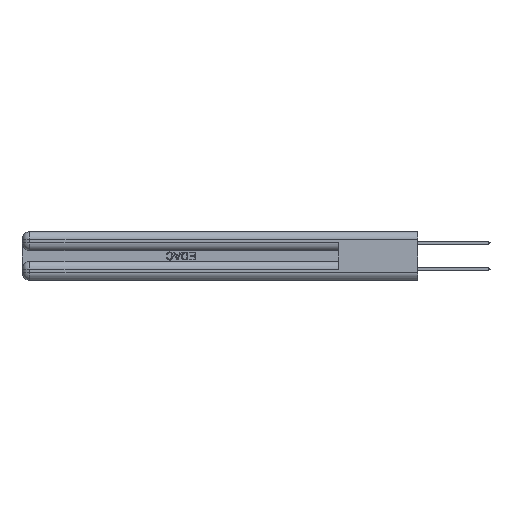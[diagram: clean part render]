
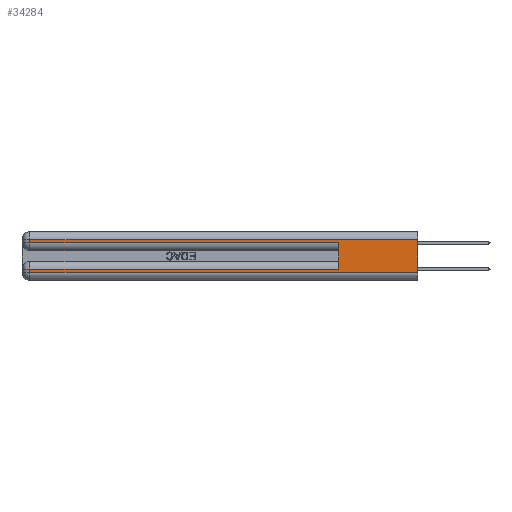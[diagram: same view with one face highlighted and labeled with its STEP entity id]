
A CAD part, left-side view. The second image highlights one B-rep face of the part: STEP entity #34284.
In plain terms, the highlighted planar face has unit normal (-1, 0, 0).
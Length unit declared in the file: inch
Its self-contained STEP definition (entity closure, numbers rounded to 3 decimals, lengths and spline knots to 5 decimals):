
#459 = DIRECTION ( 'NONE',  ( 0., 0., -1. ) ) ;
#741 = CARTESIAN_POINT ( 'NONE',  ( 0., 2.94, 0.31 ) ) ;
#1753 = DIRECTION ( 'NONE',  ( 0., -1., 0. ) ) ;
#1920 = DIRECTION ( 'NONE',  ( 0., 1., 0. ) ) ;
#2274 = VECTOR ( 'NONE', #1920, 39.37008 ) ;
#2917 = CARTESIAN_POINT ( 'NONE',  ( 0., 0., 0.31 ) ) ;
#3587 = CARTESIAN_POINT ( 'NONE',  ( 0., 0., 0.37 ) ) ;
#4552 = LINE ( 'NONE', #31151, #2274 ) ;
#6054 = VERTEX_POINT ( 'NONE', #741 ) ;
#6166 = ORIENTED_EDGE ( 'NONE', *, *, #24163, .F. ) ;
#6481 = EDGE_CURVE ( 'NONE', #37603, #10465, #30881, .T. ) ;
#7422 = VERTEX_POINT ( 'NONE', #20248 ) ;
#7532 = ORIENTED_EDGE ( 'NONE', *, *, #6481, .T. ) ;
#7965 = EDGE_CURVE ( 'NONE', #44316, #7422, #21030, .T. ) ;
#8741 = CARTESIAN_POINT ( 'NONE',  ( 0., 0., 0.06 ) ) ;
#8905 = DIRECTION ( 'NONE',  ( 0., 0., -1. ) ) ;
#9258 = ORIENTED_EDGE ( 'NONE', *, *, #30549, .T. ) ;
#10465 = VERTEX_POINT ( 'NONE', #8741 ) ;
#10579 = AXIS2_PLACEMENT_3D ( 'NONE', #35057, #38712, #16805 ) ;
#10701 = EDGE_CURVE ( 'NONE', #11947, #37603, #33867, .T. ) ;
#10733 = LINE ( 'NONE', #18638, #29027 ) ;
#11090 = DIRECTION ( 'NONE',  ( 0., -1., 0. ) ) ;
#11132 = ORIENTED_EDGE ( 'NONE', *, *, #12172, .T. ) ;
#11451 = VECTOR ( 'NONE', #11090, 39.37008 ) ;
#11481 = CARTESIAN_POINT ( 'NONE',  ( 0., 0.6, 0.085 ) ) ;
#11841 = CARTESIAN_POINT ( 'NONE',  ( 0., 2.94, 0.085 ) ) ;
#11947 = VERTEX_POINT ( 'NONE', #11841 ) ;
#11963 = CARTESIAN_POINT ( 'NONE',  ( 0., 0., 0.085 ) ) ;
#12007 = ORIENTED_EDGE ( 'NONE', *, *, #10701, .T. ) ;
#12172 = EDGE_CURVE ( 'NONE', #15923, #6054, #4552, .T. ) ;
#13122 = PLANE ( 'NONE',  #10579 ) ;
#14405 = VECTOR ( 'NONE', #35611, 39.37008 ) ;
#15923 = VERTEX_POINT ( 'NONE', #2917 ) ;
#16805 = DIRECTION ( 'NONE',  ( 0., 0., -1. ) ) ;
#18638 = CARTESIAN_POINT ( 'NONE',  ( 0., 2.94, 0.37 ) ) ;
#20248 = CARTESIAN_POINT ( 'NONE',  ( 0., 0.6, 0.285 ) ) ;
#20875 = CARTESIAN_POINT ( 'NONE',  ( 0., 0.6, 0.145 ) ) ;
#21030 = LINE ( 'NONE', #45521, #38196 ) ;
#21516 = EDGE_CURVE ( 'NONE', #15923, #10465, #21753, .T. ) ;
#21753 = LINE ( 'NONE', #3587, #30342 ) ;
#24160 = VECTOR ( 'NONE', #8905, 39.37008 ) ;
#24163 = EDGE_CURVE ( 'NONE', #34785, #7422, #33849, .T. ) ;
#25583 = VECTOR ( 'NONE', #41176, 39.37008 ) ;
#26670 = EDGE_CURVE ( 'NONE', #34785, #11947, #42744, .T. ) ;
#29027 = VECTOR ( 'NONE', #459, 39.37008 ) ;
#30342 = VECTOR ( 'NONE', #40014, 39.37008 ) ;
#30549 = EDGE_CURVE ( 'NONE', #6054, #44316, #10733, .T. ) ;
#30881 = LINE ( 'NONE', #32821, #11451 ) ;
#31151 = CARTESIAN_POINT ( 'NONE',  ( 0., 0., 0.31 ) ) ;
#32821 = CARTESIAN_POINT ( 'NONE',  ( 0., 0., 0.06 ) ) ;
#33683 = EDGE_LOOP ( 'NONE', ( #34323, #11132, #9258, #40799, #6166, #42145, #12007, #7532 ) ) ;
#33849 = LINE ( 'NONE', #20875, #14405 ) ;
#33867 = LINE ( 'NONE', #41626, #24160 ) ;
#34284 = ADVANCED_FACE ( 'NONE', ( #45817 ), #13122, .F. ) ;
#34323 = ORIENTED_EDGE ( 'NONE', *, *, #21516, .F. ) ;
#34785 = VERTEX_POINT ( 'NONE', #11481 ) ;
#35057 = CARTESIAN_POINT ( 'NONE',  ( 0., 0., 0.37 ) ) ;
#35611 = DIRECTION ( 'NONE',  ( 0., 0., 1. ) ) ;
#37603 = VERTEX_POINT ( 'NONE', #46998 ) ;
#38196 = VECTOR ( 'NONE', #1753, 39.37008 ) ;
#38712 = DIRECTION ( 'NONE',  ( 1., 0., 0. ) ) ;
#40014 = DIRECTION ( 'NONE',  ( 0., 0., -1. ) ) ;
#40799 = ORIENTED_EDGE ( 'NONE', *, *, #7965, .T. ) ;
#41176 = DIRECTION ( 'NONE',  ( 0., 1., 0. ) ) ;
#41626 = CARTESIAN_POINT ( 'NONE',  ( 0., 2.94, 0.37 ) ) ;
#42145 = ORIENTED_EDGE ( 'NONE', *, *, #26670, .T. ) ;
#42744 = LINE ( 'NONE', #11963, #25583 ) ;
#43843 = CARTESIAN_POINT ( 'NONE',  ( 0., 2.94, 0.285 ) ) ;
#44316 = VERTEX_POINT ( 'NONE', #43843 ) ;
#45521 = CARTESIAN_POINT ( 'NONE',  ( 0., 0., 0.285 ) ) ;
#45817 = FACE_OUTER_BOUND ( 'NONE', #33683, .T. ) ;
#46998 = CARTESIAN_POINT ( 'NONE',  ( 0., 2.94, 0.06 ) ) ;
